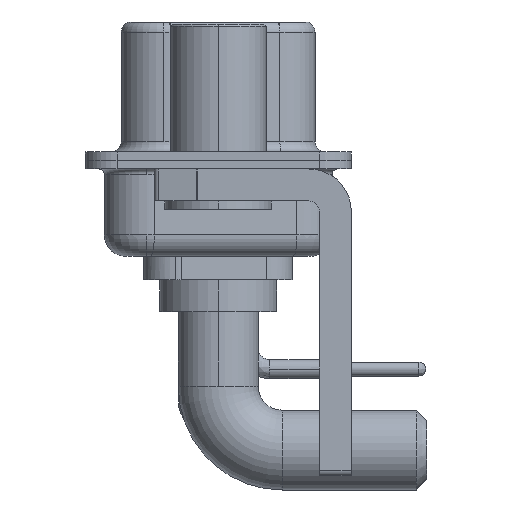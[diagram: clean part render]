
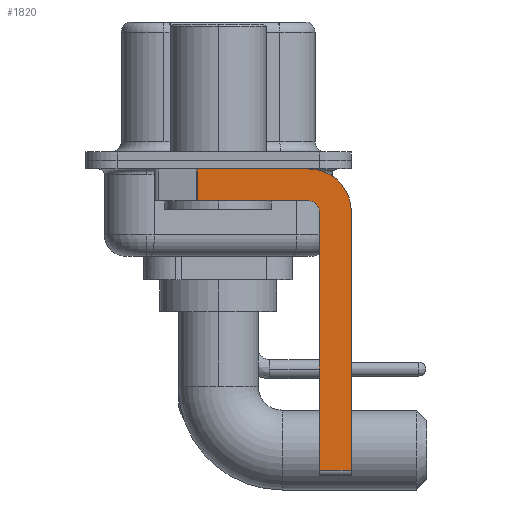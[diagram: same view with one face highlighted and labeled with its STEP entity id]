
A CAD part, left-side view. The second image highlights one B-rep face of the part: STEP entity #1820.
In plain terms, the highlighted planar face has unit normal (-1, 0, 0).
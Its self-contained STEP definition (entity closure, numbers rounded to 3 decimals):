
#155 = VERTEX_POINT ( 'NONE', #18076 ) ;
#996 = DIRECTION ( 'NONE',  ( 0., 0., -1. ) ) ;
#1194 = ORIENTED_EDGE ( 'NONE', *, *, #5038, .F. ) ;
#1457 = CARTESIAN_POINT ( 'NONE',  ( -2.9, -4.75, -14.8 ) ) ;
#1594 = CARTESIAN_POINT ( 'NONE',  ( -2.9, -6.25, -2.4 ) ) ;
#1820 = ADVANCED_FACE ( 'NONE', ( #16200 ), #14053, .F. ) ;
#2435 = CARTESIAN_POINT ( 'NONE',  ( -2.9, 0.978, -0.4 ) ) ;
#2898 = ORIENTED_EDGE ( 'NONE', *, *, #25278, .T. ) ;
#3355 = DIRECTION ( 'NONE',  ( 0., -1., 0. ) ) ;
#4157 = LINE ( 'NONE', #16174, #15263 ) ;
#5038 = EDGE_CURVE ( 'NONE', #8912, #155, #19944, .T. ) ;
#5242 = DIRECTION ( 'NONE',  ( 0., 0., -1. ) ) ;
#5667 = VERTEX_POINT ( 'NONE', #12057 ) ;
#5672 = VERTEX_POINT ( 'NONE', #18977 ) ;
#5696 = VECTOR ( 'NONE', #3355, 1000. ) ;
#6152 = DIRECTION ( 'NONE',  ( 0., 0., -1. ) ) ;
#6454 = LINE ( 'NONE', #25205, #18752 ) ;
#6901 = CARTESIAN_POINT ( 'NONE',  ( -2.9, -4.25, -1.9 ) ) ;
#7329 = ORIENTED_EDGE ( 'NONE', *, *, #23043, .F. ) ;
#7710 = CARTESIAN_POINT ( 'NONE',  ( -2.9, -4.25, -2.4 ) ) ;
#7964 = ORIENTED_EDGE ( 'NONE', *, *, #14676, .F. ) ;
#8912 = VERTEX_POINT ( 'NONE', #20351 ) ;
#9219 = ORIENTED_EDGE ( 'NONE', *, *, #15465, .F. ) ;
#9655 = ORIENTED_EDGE ( 'NONE', *, *, #26559, .F. ) ;
#9738 = CARTESIAN_POINT ( 'NONE',  ( -2.9, -4.25, -2.4 ) ) ;
#10631 = CARTESIAN_POINT ( 'NONE',  ( -2.9, 3., -0.4 ) ) ;
#11900 = AXIS2_PLACEMENT_3D ( 'NONE', #7710, #12496, #5242 ) ;
#11969 = VERTEX_POINT ( 'NONE', #29743 ) ;
#12057 = CARTESIAN_POINT ( 'NONE',  ( -2.9, 0.978, -1.9 ) ) ;
#12496 = DIRECTION ( 'NONE',  ( 1., 0., 0. ) ) ;
#14053 = PLANE ( 'NONE',  #29719 ) ;
#14676 = EDGE_CURVE ( 'NONE', #18997, #5672, #24860, .T. ) ;
#14744 = CARTESIAN_POINT ( 'NONE',  ( -2.9, -4.25, -1.9 ) ) ;
#15263 = VECTOR ( 'NONE', #25378, 1000. ) ;
#15284 = VECTOR ( 'NONE', #25659, 1000. ) ;
#15465 = EDGE_CURVE ( 'NONE', #155, #19539, #18945, .T. ) ;
#16174 = CARTESIAN_POINT ( 'NONE',  ( -2.9, -4.25, -14.55 ) ) ;
#16200 = FACE_OUTER_BOUND ( 'NONE', #26909, .T. ) ;
#16539 = EDGE_CURVE ( 'NONE', #27845, #11969, #22302, .T. ) ;
#16914 = VECTOR ( 'NONE', #996, 1000. ) ;
#17474 = VECTOR ( 'NONE', #22090, 1000. ) ;
#17760 = ORIENTED_EDGE ( 'NONE', *, *, #16539, .F. ) ;
#18076 = CARTESIAN_POINT ( 'NONE',  ( -2.9, -4.75, -2.4 ) ) ;
#18752 = VECTOR ( 'NONE', #6152, 1000. ) ;
#18945 = CIRCLE ( 'NONE', #25795, 0.5 ) ;
#18977 = CARTESIAN_POINT ( 'NONE',  ( -2.9, -6.25, -14.55 ) ) ;
#18997 = VERTEX_POINT ( 'NONE', #1594 ) ;
#19539 = VERTEX_POINT ( 'NONE', #14744 ) ;
#19944 = LINE ( 'NONE', #1457, #17474 ) ;
#20351 = CARTESIAN_POINT ( 'NONE',  ( -2.9, -4.75, -14.55 ) ) ;
#21107 = DIRECTION ( 'NONE',  ( 0., 0., -1. ) ) ;
#21913 = EDGE_CURVE ( 'NONE', #8912, #5672, #4157, .T. ) ;
#22090 = DIRECTION ( 'NONE',  ( 0., 0., 1. ) ) ;
#22095 = CARTESIAN_POINT ( 'NONE',  ( -2.9, -6.25, -2.4 ) ) ;
#22302 = LINE ( 'NONE', #10631, #5696 ) ;
#23043 = EDGE_CURVE ( 'NONE', #11969, #18997, #25125, .T. ) ;
#24012 = DIRECTION ( 'NONE',  ( 0., 0., 1. ) ) ;
#24860 = LINE ( 'NONE', #22095, #16914 ) ;
#25125 = CIRCLE ( 'NONE', #11900, 2. ) ;
#25205 = CARTESIAN_POINT ( 'NONE',  ( -2.9, 0.978, -1.9 ) ) ;
#25278 = EDGE_CURVE ( 'NONE', #27845, #5667, #6454, .T. ) ;
#25378 = DIRECTION ( 'NONE',  ( 0., -1., 0. ) ) ;
#25460 = ORIENTED_EDGE ( 'NONE', *, *, #21913, .T. ) ;
#25548 = CARTESIAN_POINT ( 'NONE',  ( -2.9, -4.25, -2.4 ) ) ;
#25659 = DIRECTION ( 'NONE',  ( 0., 1., 0. ) ) ;
#25795 = AXIS2_PLACEMENT_3D ( 'NONE', #9738, #28488, #24012 ) ;
#26559 = EDGE_CURVE ( 'NONE', #19539, #5667, #27970, .T. ) ;
#26909 = EDGE_LOOP ( 'NONE', ( #17760, #2898, #9655, #9219, #1194, #25460, #7964, #7329 ) ) ;
#27845 = VERTEX_POINT ( 'NONE', #2435 ) ;
#27970 = LINE ( 'NONE', #6901, #15284 ) ;
#28327 = DIRECTION ( 'NONE',  ( 1., 0., 0. ) ) ;
#28488 = DIRECTION ( 'NONE',  ( -1., 0., 0. ) ) ;
#29719 = AXIS2_PLACEMENT_3D ( 'NONE', #25548, #28327, #21107 ) ;
#29743 = CARTESIAN_POINT ( 'NONE',  ( -2.9, -4.25, -0.4 ) ) ;
